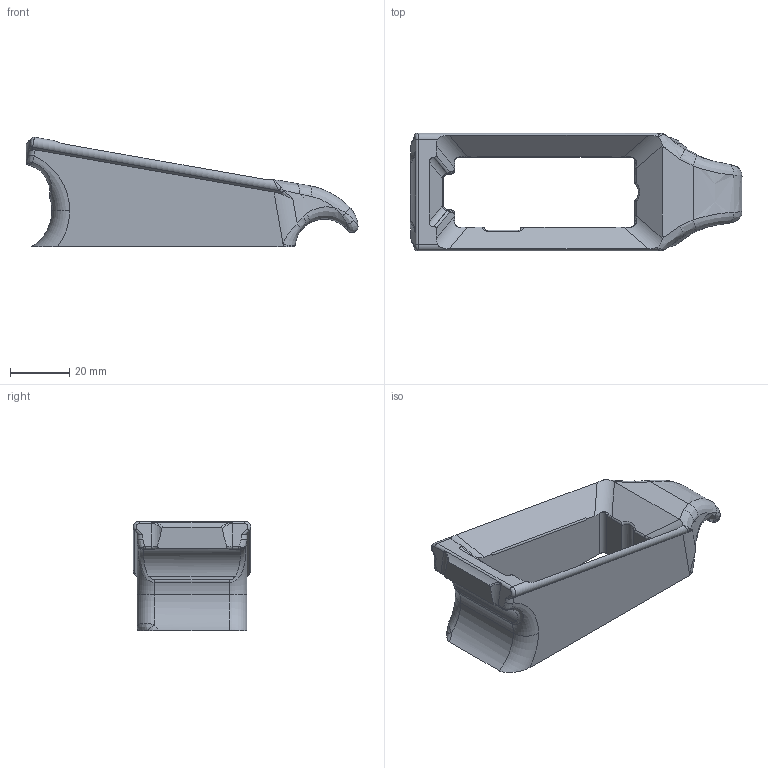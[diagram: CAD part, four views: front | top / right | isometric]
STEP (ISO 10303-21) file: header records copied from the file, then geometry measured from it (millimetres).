
FILE_DESCRIPTION (( 'STEP AP214' ), '1' );
FILE_NAME ('Magwell_3b.STEP', '2015-10-23T19:40:30', ( 'WarFairy' ), ( '' ), 'SwSTEP 2.0', 'SolidWorks 2015', '' );
FILE_SCHEMA (( 'AUTOMOTIVE_DESIGN' ));
Length unit declared in the file: inch
Products named in the file (1): Magwell_3b
Bounding box: 112.19 x 39.78 x 37.04 mm (x, y, z)
Volume: 46693.9 mm3; surface area: 16239.7 mm2
Topology: 1 solids, 1 shells, 192 faces, 514 edges, 316 vertices
Faces by surface type: bspline 81, cylinder 51, plane 46, torus 12, sphere 2
Entity records: 9477 total; most frequent: CARTESIAN_POINT 5471, ORIENTED_EDGE 1014, DIRECTION 602, EDGE_CURVE 507, VERTEX_POINT 316, AXIS2_PLACEMENT_3D 220, EDGE_LOOP 193, ADVANCED_FACE 192
